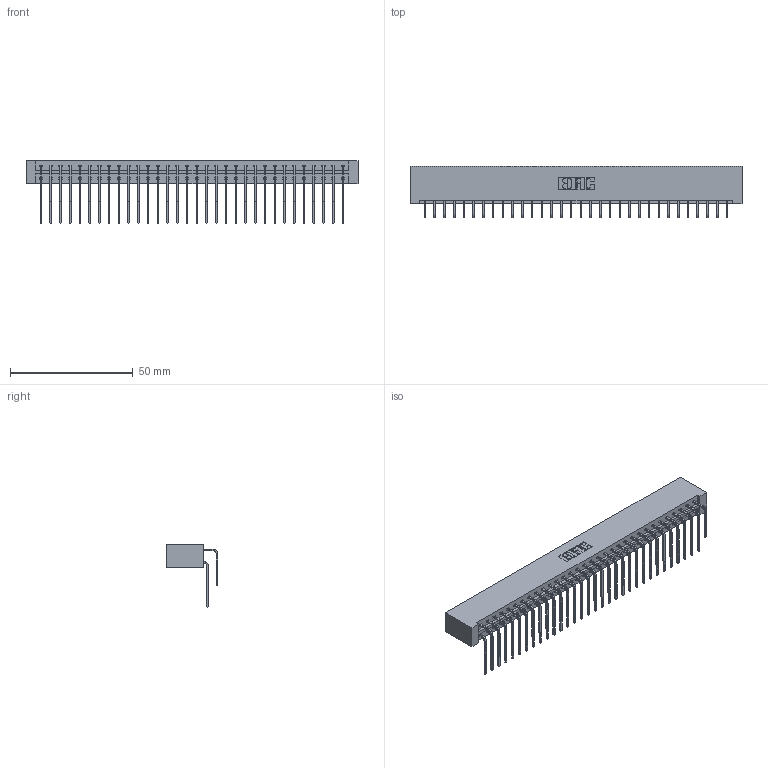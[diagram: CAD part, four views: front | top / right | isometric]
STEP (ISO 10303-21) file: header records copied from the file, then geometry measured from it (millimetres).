
FILE_DESCRIPTION (( 'STEP AP203' ), '1' );
FILE_NAME ('333-064-559-201.STEP', '2018-08-04T10:33:47', ( '' ), ( '' ), 'SwSTEP 2.0', 'SolidWorks 2016', '' );
FILE_SCHEMA (( 'CONFIG_CONTROL_DESIGN' ));
Length unit declared in the file: inch
Products named in the file (4): 333 Part_Lugless; 345-292-001_558 559 Tail - 1; 345-292-001_559 Tail - 2; 333-064-559-201
Assembly tree (65 placements, depth 2):
  333-064-559-201
    333 Part_Lugless
    345-292-001_558 559 Tail - 1  x32
    345-292-001_559 Tail - 2  x32
Bounding box: 135.05 x 20.9 x 25.53 mm (x, y, z)
Volume: 14695.9 mm3; surface area: 19130.1 mm2
Topology: 65 solids, 65 shells, 3562 faces, 10591 edges, 6974 vertices
Faces by surface type: plane 2498, cylinder 1064
Entity records: 23387 total; most frequent: CARTESIAN_POINT 3937, ORIENTED_EDGE 3822, DIRECTION 3355, EDGE_CURVE 1911, VECTOR 1751, LINE 1751, VERTEX_POINT 1270, AXIS2_PLACEMENT_3D 802
